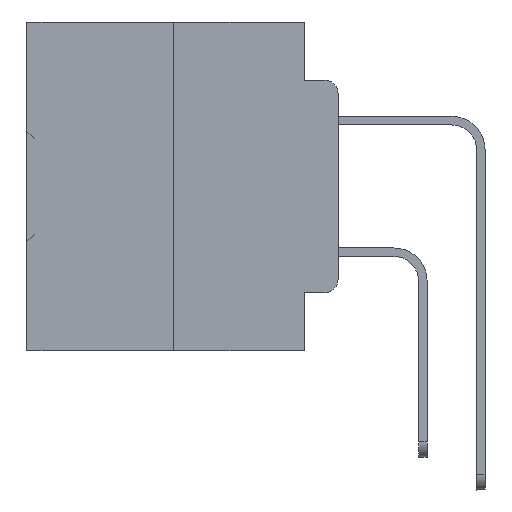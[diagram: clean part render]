
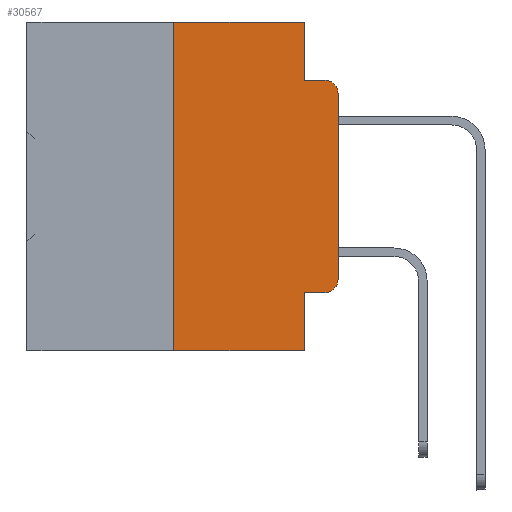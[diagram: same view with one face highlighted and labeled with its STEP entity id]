
A CAD part, left-side view. The second image highlights one B-rep face of the part: STEP entity #30567.
In plain terms, the highlighted planar face has unit normal (-1, 0, 0).
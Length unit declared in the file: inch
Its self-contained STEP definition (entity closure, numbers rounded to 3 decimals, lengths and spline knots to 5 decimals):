
#223 = ORIENTED_EDGE ( 'NONE', *, *, #4292, .F. ) ;
#421 = VERTEX_POINT ( 'NONE', #39213 ) ;
#456 = LINE ( 'NONE', #31131, #34663 ) ;
#761 = ORIENTED_EDGE ( 'NONE', *, *, #16133, .T. ) ;
#1890 = VECTOR ( 'NONE', #4511, 39.37008 ) ;
#2297 = ORIENTED_EDGE ( 'NONE', *, *, #31533, .F. ) ;
#2797 = VERTEX_POINT ( 'NONE', #37742 ) ;
#2932 = CARTESIAN_POINT ( 'NONE',  ( 0., 0., 0. ) ) ;
#3136 = DIRECTION ( 'NONE',  ( 0., -1., 0. ) ) ;
#3795 = ORIENTED_EDGE ( 'NONE', *, *, #13282, .T. ) ;
#4292 = EDGE_CURVE ( 'NONE', #28673, #421, #27348, .T. ) ;
#4511 = DIRECTION ( 'NONE',  ( 0., 0., -1. ) ) ;
#4867 = AXIS2_PLACEMENT_3D ( 'NONE', #30253, #11668, #33367 ) ;
#5488 = AXIS2_PLACEMENT_3D ( 'NONE', #31124, #12563, #34209 ) ;
#5980 = VECTOR ( 'NONE', #34610, 39.37008 ) ;
#7785 = ORIENTED_EDGE ( 'NONE', *, *, #34078, .F. ) ;
#8120 = CARTESIAN_POINT ( 'NONE',  ( 0., 0.25, 0. ) ) ;
#8691 = CARTESIAN_POINT ( 'NONE',  ( 0., 0.051, -0.0885 ) ) ;
#9290 = PLANE ( 'NONE',  #27622 ) ;
#10375 = ORIENTED_EDGE ( 'NONE', *, *, #22388, .T. ) ;
#11668 = DIRECTION ( 'NONE',  ( -1., 0., 0. ) ) ;
#12114 = VECTOR ( 'NONE', #31451, 39.37008 ) ;
#12288 = CARTESIAN_POINT ( 'NONE',  ( 0., 0.25, 0. ) ) ;
#12563 = DIRECTION ( 'NONE',  ( -1., 0., 0. ) ) ;
#12775 = DIRECTION ( 'NONE',  ( 0., -1., 0. ) ) ;
#12840 = FACE_OUTER_BOUND ( 'NONE', #18864, .T. ) ;
#13282 = EDGE_CURVE ( 'NONE', #14025, #421, #27331, .T. ) ;
#13679 = ORIENTED_EDGE ( 'NONE', *, *, #22449, .F. ) ;
#13694 = ORIENTED_EDGE ( 'NONE', *, *, #25170, .T. ) ;
#14025 = VERTEX_POINT ( 'NONE', #21424 ) ;
#14956 = CIRCLE ( 'NONE', #5488, 0.02 ) ;
#15458 = DIRECTION ( 'NONE',  ( 0., 0., 1. ) ) ;
#15536 = CARTESIAN_POINT ( 'NONE',  ( 0., 0.051, -0.4115 ) ) ;
#15635 = DIRECTION ( 'NONE',  ( 0., 0., -1. ) ) ;
#16133 = EDGE_CURVE ( 'NONE', #18376, #14025, #31405, .T. ) ;
#16412 = VECTOR ( 'NONE', #15458, 39.37008 ) ;
#18376 = VERTEX_POINT ( 'NONE', #28794 ) ;
#18413 = LINE ( 'NONE', #12288, #16412 ) ;
#18777 = LINE ( 'NONE', #26401, #1890 ) ;
#18864 = EDGE_LOOP ( 'NONE', ( #761, #3795, #223, #2297, #13679, #32244, #10375, #7785, #13694, #22590 ) ) ;
#19191 = VECTOR ( 'NONE', #26058, 39.37008 ) ;
#19906 = CARTESIAN_POINT ( 'NONE',  ( 0., 0.051, -0.0885 ) ) ;
#21424 = CARTESIAN_POINT ( 'NONE',  ( 0., 0., -0.1085 ) ) ;
#21888 = DIRECTION ( 'NONE',  ( 0., 0., 1. ) ) ;
#22145 = CARTESIAN_POINT ( 'NONE',  ( 0., 0.051, -0.4115 ) ) ;
#22388 = EDGE_CURVE ( 'NONE', #26947, #27770, #456, .T. ) ;
#22449 = EDGE_CURVE ( 'NONE', #35044, #2797, #30838, .T. ) ;
#22590 = ORIENTED_EDGE ( 'NONE', *, *, #24477, .T. ) ;
#24477 = EDGE_CURVE ( 'NONE', #38199, #18376, #14956, .T. ) ;
#24835 = CARTESIAN_POINT ( 'NONE',  ( 0., 0.25, -0.5 ) ) ;
#25170 = EDGE_CURVE ( 'NONE', #34010, #38199, #38036, .T. ) ;
#26058 = DIRECTION ( 'NONE',  ( 0., -1., 0. ) ) ;
#26401 = CARTESIAN_POINT ( 'NONE',  ( 0., 0.051, 0. ) ) ;
#26947 = VERTEX_POINT ( 'NONE', #24835 ) ;
#27331 = CIRCLE ( 'NONE', #4867, 0.02 ) ;
#27348 = LINE ( 'NONE', #19906, #19191 ) ;
#27622 = AXIS2_PLACEMENT_3D ( 'NONE', #31040, #34114, #15635 ) ;
#27770 = VERTEX_POINT ( 'NONE', #29171 ) ;
#28611 = LINE ( 'NONE', #37477, #12114 ) ;
#28673 = VERTEX_POINT ( 'NONE', #8691 ) ;
#28794 = CARTESIAN_POINT ( 'NONE',  ( 0., 0., -0.3915 ) ) ;
#29171 = CARTESIAN_POINT ( 'NONE',  ( 0., 0.051, -0.5 ) ) ;
#29316 = EDGE_CURVE ( 'NONE', #26947, #35044, #18413, .T. ) ;
#30253 = CARTESIAN_POINT ( 'NONE',  ( 0., 0.02, -0.1085 ) ) ;
#30567 = ADVANCED_FACE ( 'NONE', ( #12840 ), #9290, .F. ) ;
#30838 = LINE ( 'NONE', #31523, #5980 ) ;
#31040 = CARTESIAN_POINT ( 'NONE',  ( 0., 0.473, 0. ) ) ;
#31124 = CARTESIAN_POINT ( 'NONE',  ( 0., 0.02, -0.3915 ) ) ;
#31131 = CARTESIAN_POINT ( 'NONE',  ( 0., 0.473, -0.5 ) ) ;
#31405 = LINE ( 'NONE', #2932, #36671 ) ;
#31451 = DIRECTION ( 'NONE',  ( 0., 0., -1. ) ) ;
#31523 = CARTESIAN_POINT ( 'NONE',  ( 0., 0.473, 0. ) ) ;
#31533 = EDGE_CURVE ( 'NONE', #2797, #28673, #18777, .T. ) ;
#32244 = ORIENTED_EDGE ( 'NONE', *, *, #29316, .F. ) ;
#33367 = DIRECTION ( 'NONE',  ( 0., 0., -1. ) ) ;
#34010 = VERTEX_POINT ( 'NONE', #15536 ) ;
#34078 = EDGE_CURVE ( 'NONE', #34010, #27770, #28611, .T. ) ;
#34114 = DIRECTION ( 'NONE',  ( 1., 0., 0. ) ) ;
#34209 = DIRECTION ( 'NONE',  ( 0., 0., -1. ) ) ;
#34610 = DIRECTION ( 'NONE',  ( 0., -1., 0. ) ) ;
#34663 = VECTOR ( 'NONE', #3136, 39.37008 ) ;
#35044 = VERTEX_POINT ( 'NONE', #8120 ) ;
#36671 = VECTOR ( 'NONE', #21888, 39.37008 ) ;
#37079 = VECTOR ( 'NONE', #12775, 39.37008 ) ;
#37477 = CARTESIAN_POINT ( 'NONE',  ( 0., 0.051, 0. ) ) ;
#37742 = CARTESIAN_POINT ( 'NONE',  ( 0., 0.051, 0. ) ) ;
#38036 = LINE ( 'NONE', #22145, #37079 ) ;
#38199 = VERTEX_POINT ( 'NONE', #38671 ) ;
#38671 = CARTESIAN_POINT ( 'NONE',  ( 0., 0.02, -0.4115 ) ) ;
#39213 = CARTESIAN_POINT ( 'NONE',  ( 0., 0.02, -0.0885 ) ) ;
